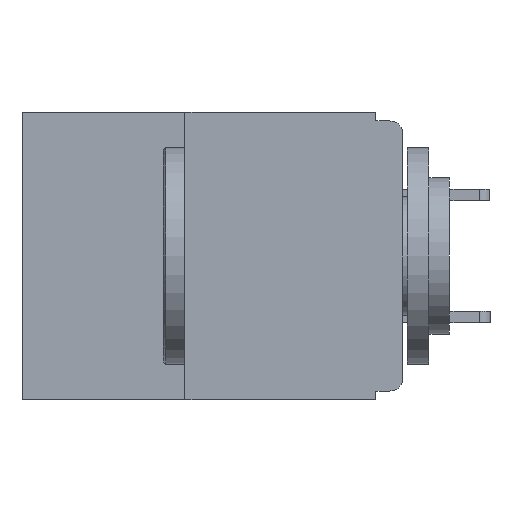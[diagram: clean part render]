
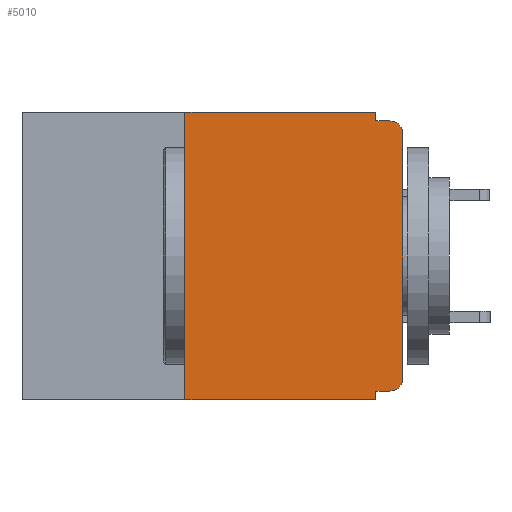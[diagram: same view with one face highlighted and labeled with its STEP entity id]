
A CAD part, left-side view. The second image highlights one B-rep face of the part: STEP entity #5010.
In plain terms, the highlighted planar face has unit normal (-1, 0, 0).
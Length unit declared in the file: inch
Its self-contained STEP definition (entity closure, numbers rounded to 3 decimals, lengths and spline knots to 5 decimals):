
#622 = CARTESIAN_POINT ( 'NONE',  ( 0., 0., -0.01 ) ) ;
#911 = CARTESIAN_POINT ( 'NONE',  ( 0., 0.031, 0. ) ) ;
#1073 = CARTESIAN_POINT ( 'NONE',  ( 0., 0.25, -0.33 ) ) ;
#1681 = EDGE_CURVE ( 'NONE', #7371, #15887, #5276, .T. ) ;
#1866 = EDGE_CURVE ( 'NONE', #29681, #12468, #25086, .T. ) ;
#2238 = EDGE_CURVE ( 'NONE', #13008, #29681, #27268, .T. ) ;
#2658 = AXIS2_PLACEMENT_3D ( 'NONE', #25117, #11101, #27463 ) ;
#2855 = VERTEX_POINT ( 'NONE', #16054 ) ;
#2992 = DIRECTION ( 'NONE',  ( 0., -1., 0. ) ) ;
#3215 = ORIENTED_EDGE ( 'NONE', *, *, #8528, .T. ) ;
#3930 = CIRCLE ( 'NONE', #2658, 0.015 ) ;
#3959 = ORIENTED_EDGE ( 'NONE', *, *, #18567, .F. ) ;
#5010 = ADVANCED_FACE ( 'NONE', ( #21431 ), #21664, .F. ) ;
#5207 = DIRECTION ( 'NONE',  ( 0., 0., -1. ) ) ;
#5276 = LINE ( 'NONE', #10535, #22534 ) ;
#5724 = CARTESIAN_POINT ( 'NONE',  ( 0., 0.031, -0.33 ) ) ;
#6502 = CARTESIAN_POINT ( 'NONE',  ( 0., 0.015, -0.32 ) ) ;
#6668 = VECTOR ( 'NONE', #2992, 39.37008 ) ;
#7371 = VERTEX_POINT ( 'NONE', #14753 ) ;
#7606 = CARTESIAN_POINT ( 'NONE',  ( 0., 0.031, -0.32 ) ) ;
#7929 = CARTESIAN_POINT ( 'NONE',  ( 0., 0., -0.305 ) ) ;
#8528 = EDGE_CURVE ( 'NONE', #2855, #22061, #14651, .T. ) ;
#9151 = LINE ( 'NONE', #911, #14671 ) ;
#9375 = DIRECTION ( 'NONE',  ( 0., 1., 0. ) ) ;
#9533 = VECTOR ( 'NONE', #15157, 39.37008 ) ;
#9889 = CARTESIAN_POINT ( 'NONE',  ( 0., 0.015, -0.01 ) ) ;
#10535 = CARTESIAN_POINT ( 'NONE',  ( 0., 0.437, 0. ) ) ;
#10539 = LINE ( 'NONE', #20671, #22262 ) ;
#10643 = ORIENTED_EDGE ( 'NONE', *, *, #21118, .T. ) ;
#11101 = DIRECTION ( 'NONE',  ( -1., 0., 0. ) ) ;
#11765 = ORIENTED_EDGE ( 'NONE', *, *, #1866, .F. ) ;
#12120 = ORIENTED_EDGE ( 'NONE', *, *, #19768, .F. ) ;
#12251 = DIRECTION ( 'NONE',  ( 0., 0., -1. ) ) ;
#12441 = VECTOR ( 'NONE', #14684, 39.37008 ) ;
#12468 = VERTEX_POINT ( 'NONE', #21023 ) ;
#12667 = VECTOR ( 'NONE', #12251, 39.37008 ) ;
#12740 = VERTEX_POINT ( 'NONE', #28947 ) ;
#13008 = VERTEX_POINT ( 'NONE', #6502 ) ;
#13155 = LINE ( 'NONE', #21650, #12441 ) ;
#13671 = CARTESIAN_POINT ( 'NONE',  ( 0., 0.015, -0.025 ) ) ;
#13681 = CARTESIAN_POINT ( 'NONE',  ( 0., 0., -0.32 ) ) ;
#13814 = AXIS2_PLACEMENT_3D ( 'NONE', #13671, #29993, #16026 ) ;
#14651 = CIRCLE ( 'NONE', #13814, 0.015 ) ;
#14670 = ORIENTED_EDGE ( 'NONE', *, *, #26960, .T. ) ;
#14671 = VECTOR ( 'NONE', #26745, 39.37008 ) ;
#14684 = DIRECTION ( 'NONE',  ( 0., -1., 0. ) ) ;
#14753 = CARTESIAN_POINT ( 'NONE',  ( 0., 0.25, 0. ) ) ;
#14769 = DIRECTION ( 'NONE',  ( 0., -1., 0. ) ) ;
#15055 = EDGE_CURVE ( 'NONE', #15887, #12740, #9151, .T. ) ;
#15157 = DIRECTION ( 'NONE',  ( 0., 0., 1. ) ) ;
#15388 = ORIENTED_EDGE ( 'NONE', *, *, #1681, .F. ) ;
#15887 = VERTEX_POINT ( 'NONE', #25308 ) ;
#16026 = DIRECTION ( 'NONE',  ( 0., 0., -1. ) ) ;
#16054 = CARTESIAN_POINT ( 'NONE',  ( 0., 0., -0.025 ) ) ;
#16680 = VERTEX_POINT ( 'NONE', #7929 ) ;
#18567 = EDGE_CURVE ( 'NONE', #12740, #22061, #25389, .T. ) ;
#18951 = EDGE_LOOP ( 'NONE', ( #14670, #3215, #3959, #20154, #15388, #12120, #20522, #11765, #27107, #10643 ) ) ;
#19038 = CARTESIAN_POINT ( 'NONE',  ( 0., 0.25, -0.33 ) ) ;
#19768 = EDGE_CURVE ( 'NONE', #24306, #7371, #21997, .T. ) ;
#20154 = ORIENTED_EDGE ( 'NONE', *, *, #15055, .F. ) ;
#20177 = DIRECTION ( 'NONE',  ( 1., 0., 0. ) ) ;
#20323 = VECTOR ( 'NONE', #9375, 39.37008 ) ;
#20522 = ORIENTED_EDGE ( 'NONE', *, *, #26026, .T. ) ;
#20671 = CARTESIAN_POINT ( 'NONE',  ( 0., 0., 0. ) ) ;
#21023 = CARTESIAN_POINT ( 'NONE',  ( 0., 0.031, -0.33 ) ) ;
#21118 = EDGE_CURVE ( 'NONE', #13008, #16680, #3930, .T. ) ;
#21431 = FACE_OUTER_BOUND ( 'NONE', #18951, .T. ) ;
#21650 = CARTESIAN_POINT ( 'NONE',  ( 0., 0.437, -0.33 ) ) ;
#21664 = PLANE ( 'NONE',  #29770 ) ;
#21997 = LINE ( 'NONE', #1073, #9533 ) ;
#22061 = VERTEX_POINT ( 'NONE', #9889 ) ;
#22262 = VECTOR ( 'NONE', #23033, 39.37008 ) ;
#22534 = VECTOR ( 'NONE', #14769, 39.37008 ) ;
#23033 = DIRECTION ( 'NONE',  ( 0., 0., 1. ) ) ;
#24306 = VERTEX_POINT ( 'NONE', #19038 ) ;
#25086 = LINE ( 'NONE', #5724, #12667 ) ;
#25117 = CARTESIAN_POINT ( 'NONE',  ( 0., 0.015, -0.305 ) ) ;
#25308 = CARTESIAN_POINT ( 'NONE',  ( 0., 0.031, 0. ) ) ;
#25389 = LINE ( 'NONE', #622, #6668 ) ;
#26026 = EDGE_CURVE ( 'NONE', #24306, #12468, #13155, .T. ) ;
#26745 = DIRECTION ( 'NONE',  ( 0., 0., -1. ) ) ;
#26960 = EDGE_CURVE ( 'NONE', #16680, #2855, #10539, .T. ) ;
#27107 = ORIENTED_EDGE ( 'NONE', *, *, #2238, .F. ) ;
#27268 = LINE ( 'NONE', #13681, #20323 ) ;
#27463 = DIRECTION ( 'NONE',  ( 0., 0., -1. ) ) ;
#28347 = CARTESIAN_POINT ( 'NONE',  ( 0., 0.437, 0. ) ) ;
#28947 = CARTESIAN_POINT ( 'NONE',  ( 0., 0.031, -0.01 ) ) ;
#29681 = VERTEX_POINT ( 'NONE', #7606 ) ;
#29770 = AXIS2_PLACEMENT_3D ( 'NONE', #28347, #20177, #5207 ) ;
#29993 = DIRECTION ( 'NONE',  ( -1., 0., 0. ) ) ;
